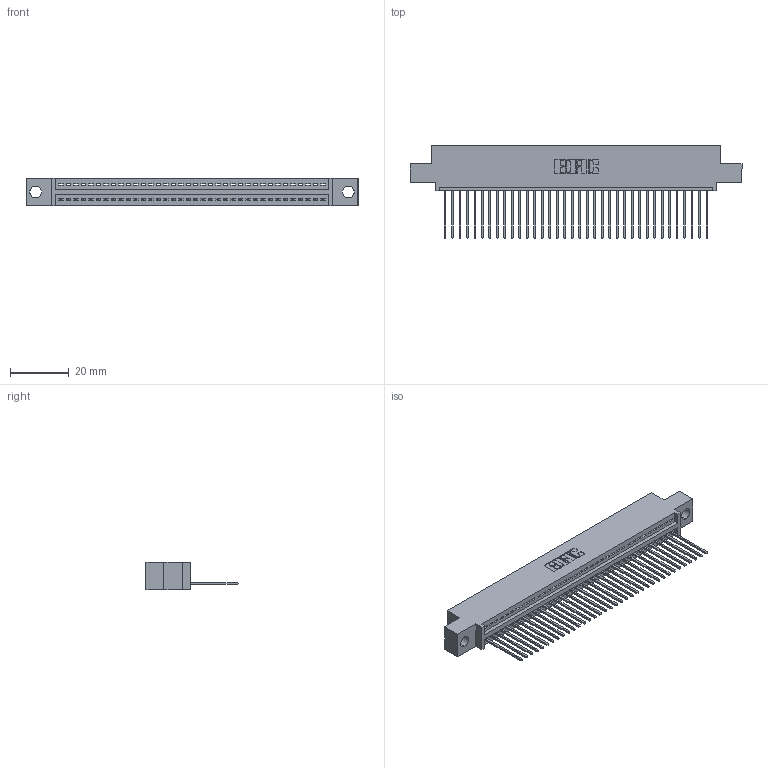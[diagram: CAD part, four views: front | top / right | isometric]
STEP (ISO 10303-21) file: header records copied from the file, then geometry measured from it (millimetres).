
FILE_DESCRIPTION (( 'STEP AP203' ), '1' );
FILE_NAME ('395-036-542-404.STEP', '2021-05-31T14:54:22', ( '' ), ( '' ), 'SwSTEP 2.0', 'SolidWorks 2020', '' );
FILE_SCHEMA (( 'CONFIG_CONTROL_DESIGN' ));
Length unit declared in the file: inch
Products named in the file (3): 345-292-001_345-293-142; 345 Part_0.110 Offset - 0.156 Dia-TI; 395-036-542-404
Assembly tree (37 placements, depth 2):
  395-036-542-404
    345 Part_0.110 Offset - 0.156 Dia-TI
    345-292-001_345-293-142  x36
Bounding box: 112.65 x 31.29 x 9.4 mm (x, y, z)
Volume: 10551.1 mm3; surface area: 14370.9 mm2
Topology: 37 solids, 37 shells, 2232 faces, 6725 edges, 4434 vertices
Faces by surface type: plane 1538, cylinder 694
Entity records: 28471 total; most frequent: CARTESIAN_POINT 4942, ORIENTED_EDGE 4910, DIRECTION 4323, EDGE_CURVE 2455, LINE 2179, VECTOR 2179, VERTEX_POINT 1634, AXIS2_PLACEMENT_3D 1072
